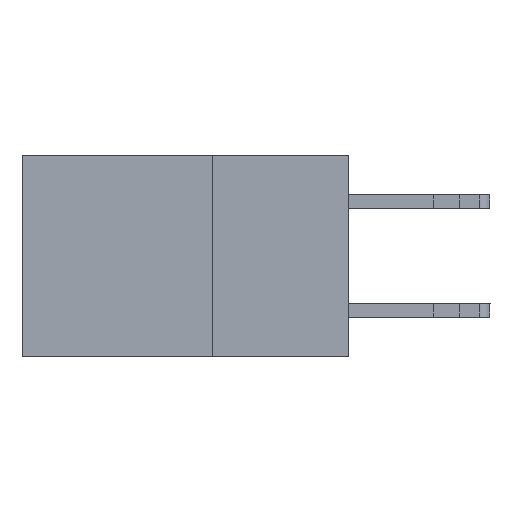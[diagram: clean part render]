
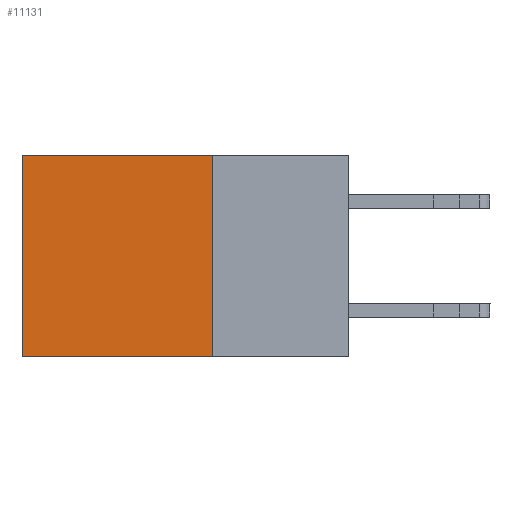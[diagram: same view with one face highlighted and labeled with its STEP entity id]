
A CAD part, left-side view. The second image highlights one B-rep face of the part: STEP entity #11131.
In plain terms, the highlighted planar face has unit normal (-1, 0, 0).
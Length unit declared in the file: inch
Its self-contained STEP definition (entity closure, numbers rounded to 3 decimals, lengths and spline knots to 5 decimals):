
#93 = CARTESIAN_POINT ( 'NONE',  ( 0.298, 0.25, -0.37 ) ) ;
#104 = CARTESIAN_POINT ( 'NONE',  ( 0.298, 0.6, 0. ) ) ;
#632 = PLANE ( 'NONE',  #15367 ) ;
#656 = ORIENTED_EDGE ( 'NONE', *, *, #18604, .F. ) ;
#1694 = EDGE_CURVE ( 'NONE', #20597, #2391, #8338, .T. ) ;
#1754 = VERTEX_POINT ( 'NONE', #16505 ) ;
#2015 = DIRECTION ( 'NONE',  ( 0., 1., 0. ) ) ;
#2391 = VERTEX_POINT ( 'NONE', #12808 ) ;
#3408 = ORIENTED_EDGE ( 'NONE', *, *, #1694, .F. ) ;
#3456 = DIRECTION ( 'NONE',  ( 0., 0., -1. ) ) ;
#3610 = CARTESIAN_POINT ( 'NONE',  ( 0.298, 0.25, -0.37 ) ) ;
#3871 = VECTOR ( 'NONE', #19862, 39.37008 ) ;
#5164 = VECTOR ( 'NONE', #2015, 39.37008 ) ;
#6119 = ORIENTED_EDGE ( 'NONE', *, *, #12636, .T. ) ;
#7890 = CARTESIAN_POINT ( 'NONE',  ( 0.298, 0.25, 0. ) ) ;
#8338 = LINE ( 'NONE', #3610, #3871 ) ;
#8371 = CARTESIAN_POINT ( 'NONE',  ( 0.298, 0.25, 0. ) ) ;
#8572 = FACE_OUTER_BOUND ( 'NONE', #15607, .T. ) ;
#10311 = DIRECTION ( 'NONE',  ( 1., 0., 0. ) ) ;
#11131 = ADVANCED_FACE ( 'NONE', ( #8572 ), #632, .F. ) ;
#11286 = DIRECTION ( 'NONE',  ( 0., 0., -1. ) ) ;
#11289 = CARTESIAN_POINT ( 'NONE',  ( 0.298, 0.25, 0. ) ) ;
#11852 = CARTESIAN_POINT ( 'NONE',  ( 0.298, 0.25, 0. ) ) ;
#12024 = VECTOR ( 'NONE', #3456, 39.37008 ) ;
#12293 = ORIENTED_EDGE ( 'NONE', *, *, #14347, .T. ) ;
#12636 = EDGE_CURVE ( 'NONE', #1754, #2391, #15575, .T. ) ;
#12808 = CARTESIAN_POINT ( 'NONE',  ( 0.298, 0.6, -0.37 ) ) ;
#12902 = LINE ( 'NONE', #8371, #5164 ) ;
#13224 = VECTOR ( 'NONE', #11286, 39.37008 ) ;
#13547 = DIRECTION ( 'NONE',  ( 0., 0., -1. ) ) ;
#14347 = EDGE_CURVE ( 'NONE', #19433, #1754, #12902, .T. ) ;
#14989 = LINE ( 'NONE', #7890, #13224 ) ;
#15367 = AXIS2_PLACEMENT_3D ( 'NONE', #11852, #10311, #13547 ) ;
#15575 = LINE ( 'NONE', #104, #12024 ) ;
#15607 = EDGE_LOOP ( 'NONE', ( #6119, #3408, #656, #12293 ) ) ;
#16505 = CARTESIAN_POINT ( 'NONE',  ( 0.298, 0.6, 0. ) ) ;
#18604 = EDGE_CURVE ( 'NONE', #19433, #20597, #14989, .T. ) ;
#19433 = VERTEX_POINT ( 'NONE', #11289 ) ;
#19862 = DIRECTION ( 'NONE',  ( 0., 1., 0. ) ) ;
#20597 = VERTEX_POINT ( 'NONE', #93 ) ;
